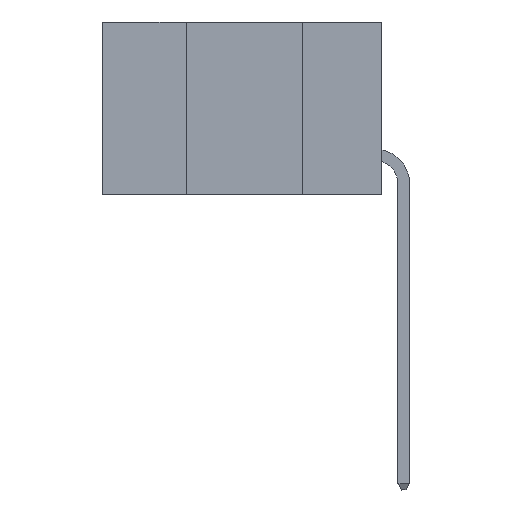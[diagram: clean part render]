
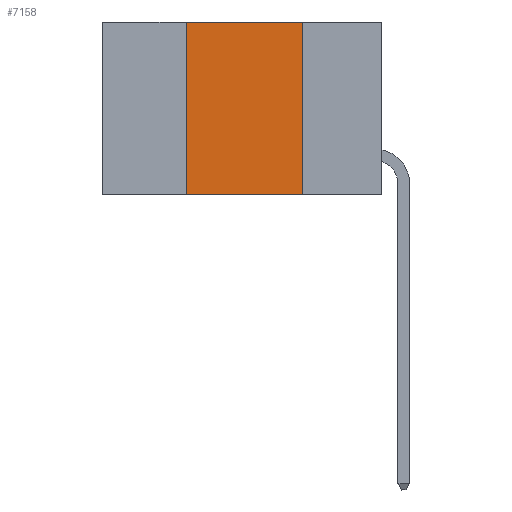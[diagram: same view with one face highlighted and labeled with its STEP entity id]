
A CAD part, left-side view. The second image highlights one B-rep face of the part: STEP entity #7158.
In plain terms, the highlighted planar face has unit normal (-1, 0, 0).
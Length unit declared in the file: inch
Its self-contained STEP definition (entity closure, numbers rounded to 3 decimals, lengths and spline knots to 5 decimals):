
#983 = EDGE_CURVE ( 'NONE', #16114, #10044, #11800, .T. ) ;
#1427 = CARTESIAN_POINT ( 'NONE',  ( 0., 0.17, 0. ) ) ;
#1494 = CARTESIAN_POINT ( 'NONE',  ( 0., 0.42, -0.37 ) ) ;
#1593 = ORIENTED_EDGE ( 'NONE', *, *, #9839, .F. ) ;
#2128 = DIRECTION ( 'NONE',  ( 0., -1., 0. ) ) ;
#2897 = VECTOR ( 'NONE', #16752, 39.37008 ) ;
#3638 = ORIENTED_EDGE ( 'NONE', *, *, #22451, .F. ) ;
#4851 = VECTOR ( 'NONE', #13466, 39.37008 ) ;
#5176 = ORIENTED_EDGE ( 'NONE', *, *, #983, .F. ) ;
#7158 = ADVANCED_FACE ( 'NONE', ( #19691 ), #20594, .F. ) ;
#8448 = CARTESIAN_POINT ( 'NONE',  ( 0., 0.42, 0. ) ) ;
#9839 = EDGE_CURVE ( 'NONE', #13304, #16864, #16568, .T. ) ;
#10044 = VERTEX_POINT ( 'NONE', #20016 ) ;
#10205 = ORIENTED_EDGE ( 'NONE', *, *, #17554, .T. ) ;
#10285 = DIRECTION ( 'NONE',  ( 1., 0., 0. ) ) ;
#11800 = LINE ( 'NONE', #1427, #19679 ) ;
#13304 = VERTEX_POINT ( 'NONE', #1494 ) ;
#13466 = DIRECTION ( 'NONE',  ( 0., 0., 1. ) ) ;
#13571 = CARTESIAN_POINT ( 'NONE',  ( 0., 0.6, 0. ) ) ;
#14230 = CARTESIAN_POINT ( 'NONE',  ( 0., 0.17, 0. ) ) ;
#15552 = DIRECTION ( 'NONE',  ( 0., 0., -1. ) ) ;
#16114 = VERTEX_POINT ( 'NONE', #14230 ) ;
#16395 = VECTOR ( 'NONE', #2128, 39.37008 ) ;
#16568 = LINE ( 'NONE', #8448, #4851 ) ;
#16752 = DIRECTION ( 'NONE',  ( 0., -1., 0. ) ) ;
#16864 = VERTEX_POINT ( 'NONE', #21517 ) ;
#17203 = DIRECTION ( 'NONE',  ( 0., 0., -1. ) ) ;
#17554 = EDGE_CURVE ( 'NONE', #13304, #10044, #19763, .T. ) ;
#19679 = VECTOR ( 'NONE', #15552, 39.37008 ) ;
#19691 = FACE_OUTER_BOUND ( 'NONE', #22360, .T. ) ;
#19763 = LINE ( 'NONE', #20292, #2897 ) ;
#19898 = LINE ( 'NONE', #21211, #16395 ) ;
#20016 = CARTESIAN_POINT ( 'NONE',  ( 0., 0.17, -0.37 ) ) ;
#20292 = CARTESIAN_POINT ( 'NONE',  ( 0., 0.6, -0.37 ) ) ;
#20594 = PLANE ( 'NONE',  #22050 ) ;
#21211 = CARTESIAN_POINT ( 'NONE',  ( 0., 0.6, 0. ) ) ;
#21517 = CARTESIAN_POINT ( 'NONE',  ( 0., 0.42, 0. ) ) ;
#22050 = AXIS2_PLACEMENT_3D ( 'NONE', #13571, #10285, #17203 ) ;
#22360 = EDGE_LOOP ( 'NONE', ( #5176, #3638, #1593, #10205 ) ) ;
#22451 = EDGE_CURVE ( 'NONE', #16864, #16114, #19898, .T. ) ;
